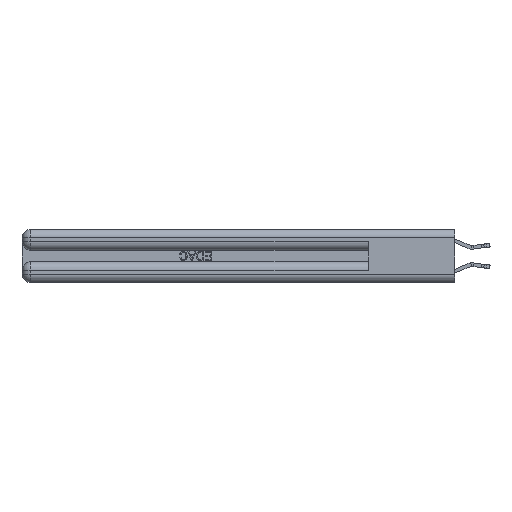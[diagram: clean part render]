
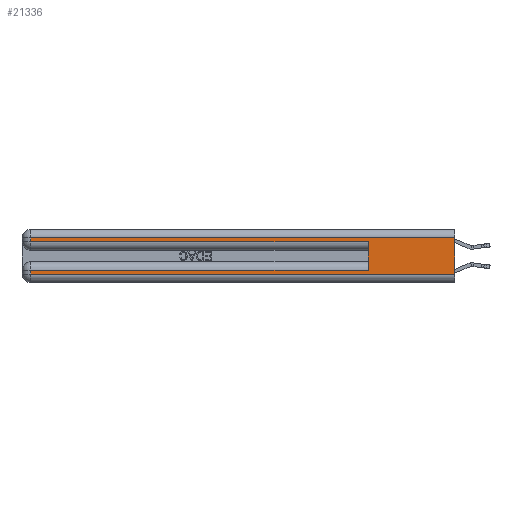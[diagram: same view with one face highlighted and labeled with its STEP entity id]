
A CAD part, left-side view. The second image highlights one B-rep face of the part: STEP entity #21336.
In plain terms, the highlighted planar face has unit normal (-1, 0, 0).
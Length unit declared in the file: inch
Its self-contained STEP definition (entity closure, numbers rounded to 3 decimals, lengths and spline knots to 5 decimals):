
#770 = LINE ( 'NONE', #24627, #7643 ) ;
#1426 = CARTESIAN_POINT ( 'NONE',  ( 0., 2.94, 0.06 ) ) ;
#1656 = VERTEX_POINT ( 'NONE', #1426 ) ;
#2486 = LINE ( 'NONE', #23576, #30478 ) ;
#3564 = CARTESIAN_POINT ( 'NONE',  ( 0., 0., 0.06 ) ) ;
#4196 = ORIENTED_EDGE ( 'NONE', *, *, #23357, .F. ) ;
#4671 = DIRECTION ( 'NONE',  ( 0., 1., 0. ) ) ;
#4713 = CARTESIAN_POINT ( 'NONE',  ( 0., 2.94, 0.31 ) ) ;
#4788 = CARTESIAN_POINT ( 'NONE',  ( 0., 0.6, 0.285 ) ) ;
#5611 = EDGE_CURVE ( 'NONE', #22985, #20811, #26447, .T. ) ;
#5676 = LINE ( 'NONE', #23689, #17783 ) ;
#6654 = DIRECTION ( 'NONE',  ( 1., 0., 0. ) ) ;
#7162 = PLANE ( 'NONE',  #33302 ) ;
#7200 = ORIENTED_EDGE ( 'NONE', *, *, #14677, .T. ) ;
#7643 = VECTOR ( 'NONE', #11237, 39.37008 ) ;
#7973 = VERTEX_POINT ( 'NONE', #3564 ) ;
#8840 = CARTESIAN_POINT ( 'NONE',  ( 0., 2.94, 0.285 ) ) ;
#10057 = FACE_OUTER_BOUND ( 'NONE', #32708, .T. ) ;
#10201 = CARTESIAN_POINT ( 'NONE',  ( 0., 0.6, 0.085 ) ) ;
#10816 = CARTESIAN_POINT ( 'NONE',  ( 0., 2.94, 0.37 ) ) ;
#11237 = DIRECTION ( 'NONE',  ( 0., 0., -1. ) ) ;
#11352 = CARTESIAN_POINT ( 'NONE',  ( 0., 2.94, 0.085 ) ) ;
#12126 = CARTESIAN_POINT ( 'NONE',  ( 0., 0., 0.37 ) ) ;
#12213 = CARTESIAN_POINT ( 'NONE',  ( 0., 0., 0.31 ) ) ;
#12320 = VERTEX_POINT ( 'NONE', #26008 ) ;
#12406 = VECTOR ( 'NONE', #33663, 39.37008 ) ;
#12451 = DIRECTION ( 'NONE',  ( 0., 0., -1. ) ) ;
#13052 = ORIENTED_EDGE ( 'NONE', *, *, #14679, .T. ) ;
#14677 = EDGE_CURVE ( 'NONE', #16736, #1656, #21122, .T. ) ;
#14679 = EDGE_CURVE ( 'NONE', #24684, #16736, #5676, .T. ) ;
#15681 = DIRECTION ( 'NONE',  ( 0., 0., 1. ) ) ;
#15999 = CARTESIAN_POINT ( 'NONE',  ( 0., 0., 0.37 ) ) ;
#16486 = VERTEX_POINT ( 'NONE', #4713 ) ;
#16736 = VERTEX_POINT ( 'NONE', #11352 ) ;
#17783 = VECTOR ( 'NONE', #20956, 39.37008 ) ;
#19049 = EDGE_CURVE ( 'NONE', #24684, #20811, #2486, .T. ) ;
#19582 = EDGE_CURVE ( 'NONE', #1656, #7973, #23032, .T. ) ;
#20292 = ORIENTED_EDGE ( 'NONE', *, *, #5611, .T. ) ;
#20514 = ORIENTED_EDGE ( 'NONE', *, *, #19049, .F. ) ;
#20811 = VERTEX_POINT ( 'NONE', #4788 ) ;
#20837 = ORIENTED_EDGE ( 'NONE', *, *, #24380, .T. ) ;
#20956 = DIRECTION ( 'NONE',  ( 0., 1., 0. ) ) ;
#21122 = LINE ( 'NONE', #10816, #25440 ) ;
#21336 = ADVANCED_FACE ( 'NONE', ( #10057 ), #7162, .F. ) ;
#22663 = ORIENTED_EDGE ( 'NONE', *, *, #19582, .T. ) ;
#22985 = VERTEX_POINT ( 'NONE', #8840 ) ;
#23032 = LINE ( 'NONE', #33495, #12406 ) ;
#23357 = EDGE_CURVE ( 'NONE', #12320, #7973, #31618, .T. ) ;
#23576 = CARTESIAN_POINT ( 'NONE',  ( 0., 0.6, 0.145 ) ) ;
#23689 = CARTESIAN_POINT ( 'NONE',  ( 0., 0., 0.085 ) ) ;
#24380 = EDGE_CURVE ( 'NONE', #16486, #22985, #770, .T. ) ;
#24627 = CARTESIAN_POINT ( 'NONE',  ( 0., 2.94, 0.37 ) ) ;
#24637 = VECTOR ( 'NONE', #33859, 39.37008 ) ;
#24684 = VERTEX_POINT ( 'NONE', #10201 ) ;
#25440 = VECTOR ( 'NONE', #26267, 39.37008 ) ;
#26008 = CARTESIAN_POINT ( 'NONE',  ( 0., 0., 0.31 ) ) ;
#26267 = DIRECTION ( 'NONE',  ( 0., 0., -1. ) ) ;
#26447 = LINE ( 'NONE', #33843, #27306 ) ;
#27306 = VECTOR ( 'NONE', #28857, 39.37008 ) ;
#28857 = DIRECTION ( 'NONE',  ( 0., -1., 0. ) ) ;
#29259 = VECTOR ( 'NONE', #4671, 39.37008 ) ;
#30247 = LINE ( 'NONE', #12213, #29259 ) ;
#30478 = VECTOR ( 'NONE', #15681, 39.37008 ) ;
#31618 = LINE ( 'NONE', #15999, #24637 ) ;
#32015 = EDGE_CURVE ( 'NONE', #12320, #16486, #30247, .T. ) ;
#32708 = EDGE_LOOP ( 'NONE', ( #4196, #33478, #20837, #20292, #20514, #13052, #7200, #22663 ) ) ;
#33302 = AXIS2_PLACEMENT_3D ( 'NONE', #12126, #6654, #12451 ) ;
#33478 = ORIENTED_EDGE ( 'NONE', *, *, #32015, .T. ) ;
#33495 = CARTESIAN_POINT ( 'NONE',  ( 0., 0., 0.06 ) ) ;
#33663 = DIRECTION ( 'NONE',  ( 0., -1., 0. ) ) ;
#33843 = CARTESIAN_POINT ( 'NONE',  ( 0., 0., 0.285 ) ) ;
#33859 = DIRECTION ( 'NONE',  ( 0., 0., -1. ) ) ;
